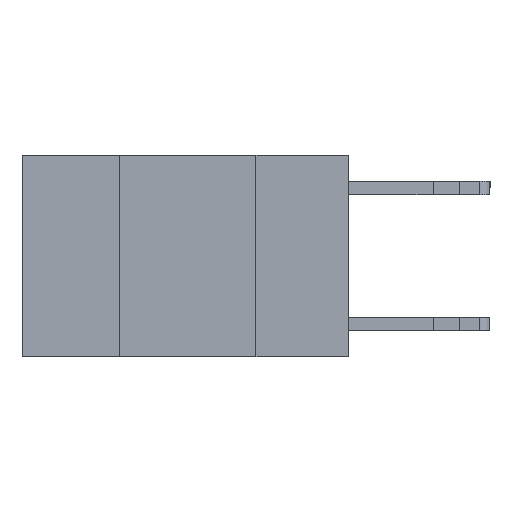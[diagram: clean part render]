
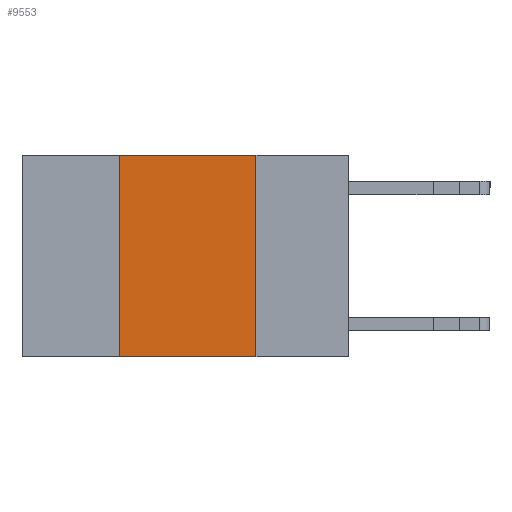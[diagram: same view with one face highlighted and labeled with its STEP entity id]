
A CAD part, left-side view. The second image highlights one B-rep face of the part: STEP entity #9553.
In plain terms, the highlighted planar face has unit normal (-1, 0, 0).
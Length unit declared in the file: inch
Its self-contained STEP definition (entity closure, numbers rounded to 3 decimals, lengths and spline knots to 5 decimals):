
#96 = EDGE_CURVE ( 'NONE', #2173, #21165, #20617, .T. ) ;
#248 = DIRECTION ( 'NONE',  ( 0., 0., -1. ) ) ;
#395 = LINE ( 'NONE', #9015, #11916 ) ;
#405 = CARTESIAN_POINT ( 'NONE',  ( 0., 0.42, -0.37 ) ) ;
#1955 = CARTESIAN_POINT ( 'NONE',  ( 0., 0.6, 0. ) ) ;
#2173 = VERTEX_POINT ( 'NONE', #4619 ) ;
#3129 = DIRECTION ( 'NONE',  ( 0., -1., 0. ) ) ;
#3746 = CARTESIAN_POINT ( 'NONE',  ( 0., 0.17, -0.37 ) ) ;
#3900 = EDGE_CURVE ( 'NONE', #7263, #17145, #395, .T. ) ;
#4335 = LINE ( 'NONE', #11199, #11077 ) ;
#4619 = CARTESIAN_POINT ( 'NONE',  ( 0., 0.17, 0. ) ) ;
#4898 = ORIENTED_EDGE ( 'NONE', *, *, #3900, .F. ) ;
#4911 = EDGE_LOOP ( 'NONE', ( #11474, #18247, #4898, #10362 ) ) ;
#5117 = CARTESIAN_POINT ( 'NONE',  ( 0., 0.17, 0. ) ) ;
#5558 = DIRECTION ( 'NONE',  ( 0., 0., -1. ) ) ;
#6212 = EDGE_CURVE ( 'NONE', #17145, #2173, #15326, .T. ) ;
#7263 = VERTEX_POINT ( 'NONE', #405 ) ;
#7437 = DIRECTION ( 'NONE',  ( 0., 0., 1. ) ) ;
#9015 = CARTESIAN_POINT ( 'NONE',  ( 0., 0.42, 0. ) ) ;
#9553 = ADVANCED_FACE ( 'NONE', ( #12124 ), #19043, .F. ) ;
#10362 = ORIENTED_EDGE ( 'NONE', *, *, #10386, .T. ) ;
#10386 = EDGE_CURVE ( 'NONE', #7263, #21165, #4335, .T. ) ;
#11077 = VECTOR ( 'NONE', #20282, 39.37008 ) ;
#11199 = CARTESIAN_POINT ( 'NONE',  ( 0., 0.6, -0.37 ) ) ;
#11474 = ORIENTED_EDGE ( 'NONE', *, *, #96, .F. ) ;
#11916 = VECTOR ( 'NONE', #7437, 39.37008 ) ;
#12124 = FACE_OUTER_BOUND ( 'NONE', #4911, .T. ) ;
#12786 = VECTOR ( 'NONE', #3129, 39.37008 ) ;
#13707 = DIRECTION ( 'NONE',  ( 1., 0., 0. ) ) ;
#15326 = LINE ( 'NONE', #18720, #12786 ) ;
#15479 = AXIS2_PLACEMENT_3D ( 'NONE', #1955, #13707, #248 ) ;
#17145 = VERTEX_POINT ( 'NONE', #17564 ) ;
#17564 = CARTESIAN_POINT ( 'NONE',  ( 0., 0.42, 0. ) ) ;
#18247 = ORIENTED_EDGE ( 'NONE', *, *, #6212, .F. ) ;
#18720 = CARTESIAN_POINT ( 'NONE',  ( 0., 0.6, 0. ) ) ;
#19043 = PLANE ( 'NONE',  #15479 ) ;
#19889 = VECTOR ( 'NONE', #5558, 39.37008 ) ;
#20282 = DIRECTION ( 'NONE',  ( 0., -1., 0. ) ) ;
#20617 = LINE ( 'NONE', #5117, #19889 ) ;
#21165 = VERTEX_POINT ( 'NONE', #3746 ) ;
